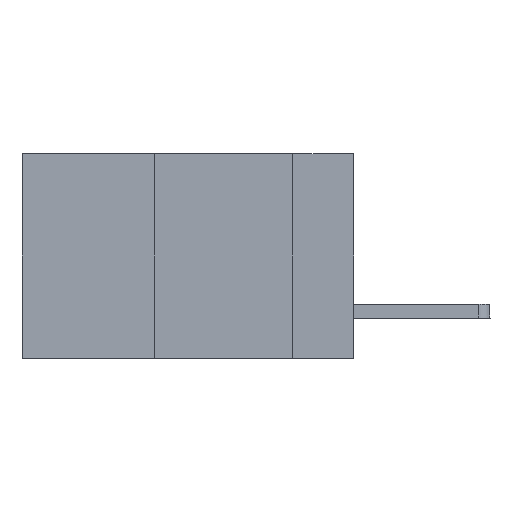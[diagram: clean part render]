
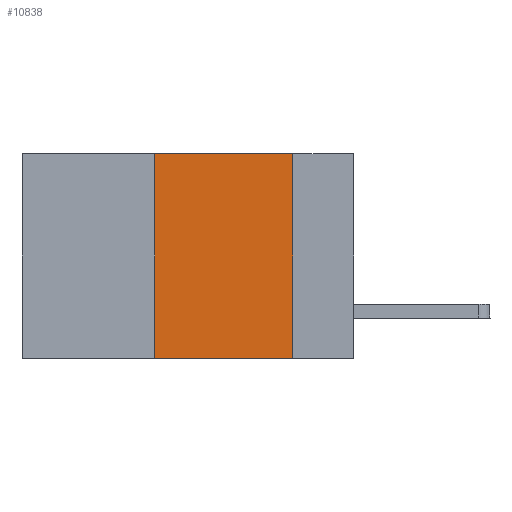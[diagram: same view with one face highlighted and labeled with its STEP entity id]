
A CAD part, left-side view. The second image highlights one B-rep face of the part: STEP entity #10838.
In plain terms, the highlighted planar face has unit normal (-1, 0, 0).
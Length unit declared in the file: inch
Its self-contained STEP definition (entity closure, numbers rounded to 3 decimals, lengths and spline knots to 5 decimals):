
#371 = LINE ( 'NONE', #656, #2761 ) ;
#656 = CARTESIAN_POINT ( 'NONE',  ( 0., 0.6, -0.37 ) ) ;
#680 = VERTEX_POINT ( 'NONE', #7867 ) ;
#778 = CARTESIAN_POINT ( 'NONE',  ( 0., 0.11, 0. ) ) ;
#1185 = EDGE_LOOP ( 'NONE', ( #9037, #9353, #1789, #8886 ) ) ;
#1568 = PLANE ( 'NONE',  #8946 ) ;
#1789 = ORIENTED_EDGE ( 'NONE', *, *, #6638, .F. ) ;
#2439 = LINE ( 'NONE', #8980, #5223 ) ;
#2574 = DIRECTION ( 'NONE',  ( 1., 0., 0. ) ) ;
#2761 = VECTOR ( 'NONE', #10767, 39.37008 ) ;
#2829 = EDGE_CURVE ( 'NONE', #3916, #10511, #11893, .T. ) ;
#3024 = FACE_OUTER_BOUND ( 'NONE', #1185, .T. ) ;
#3916 = VERTEX_POINT ( 'NONE', #6262 ) ;
#5179 = DIRECTION ( 'NONE',  ( 0., -1., 0. ) ) ;
#5223 = VECTOR ( 'NONE', #7280, 39.37008 ) ;
#5466 = CARTESIAN_POINT ( 'NONE',  ( 0., 0.6, 0. ) ) ;
#6078 = VERTEX_POINT ( 'NONE', #11918 ) ;
#6262 = CARTESIAN_POINT ( 'NONE',  ( 0., 0.36, 0. ) ) ;
#6607 = EDGE_CURVE ( 'NONE', #6078, #680, #371, .T. ) ;
#6638 = EDGE_CURVE ( 'NONE', #6078, #3916, #2439, .T. ) ;
#7280 = DIRECTION ( 'NONE',  ( 0., 0., 1. ) ) ;
#7291 = VECTOR ( 'NONE', #5179, 39.37008 ) ;
#7867 = CARTESIAN_POINT ( 'NONE',  ( 0., 0.11, -0.37 ) ) ;
#8124 = CARTESIAN_POINT ( 'NONE',  ( 0., 0.6, 0. ) ) ;
#8227 = VECTOR ( 'NONE', #9246, 39.37008 ) ;
#8886 = ORIENTED_EDGE ( 'NONE', *, *, #6607, .T. ) ;
#8946 = AXIS2_PLACEMENT_3D ( 'NONE', #8124, #2574, #9031 ) ;
#8980 = CARTESIAN_POINT ( 'NONE',  ( 0., 0.36, 0. ) ) ;
#9031 = DIRECTION ( 'NONE',  ( 0., 0., -1. ) ) ;
#9037 = ORIENTED_EDGE ( 'NONE', *, *, #10377, .F. ) ;
#9246 = DIRECTION ( 'NONE',  ( 0., 0., -1. ) ) ;
#9353 = ORIENTED_EDGE ( 'NONE', *, *, #2829, .F. ) ;
#10317 = CARTESIAN_POINT ( 'NONE',  ( 0., 0.11, 0. ) ) ;
#10377 = EDGE_CURVE ( 'NONE', #10511, #680, #10582, .T. ) ;
#10511 = VERTEX_POINT ( 'NONE', #10317 ) ;
#10582 = LINE ( 'NONE', #778, #8227 ) ;
#10767 = DIRECTION ( 'NONE',  ( 0., -1., 0. ) ) ;
#10838 = ADVANCED_FACE ( 'NONE', ( #3024 ), #1568, .F. ) ;
#11893 = LINE ( 'NONE', #5466, #7291 ) ;
#11918 = CARTESIAN_POINT ( 'NONE',  ( 0., 0.36, -0.37 ) ) ;
